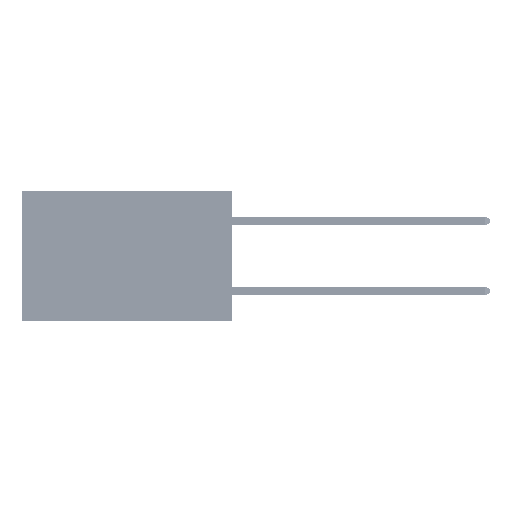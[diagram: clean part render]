
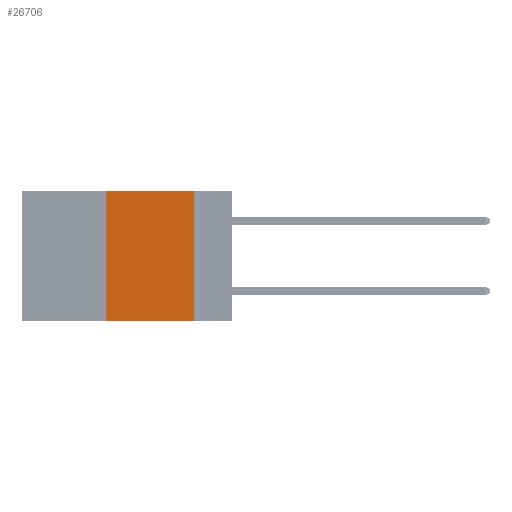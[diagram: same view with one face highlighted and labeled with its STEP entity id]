
A CAD part, left-side view. The second image highlights one B-rep face of the part: STEP entity #26706.
In plain terms, the highlighted planar face has unit normal (-1, 0, 0).
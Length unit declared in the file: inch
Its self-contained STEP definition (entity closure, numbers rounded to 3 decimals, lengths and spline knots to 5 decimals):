
#511 = CARTESIAN_POINT ( 'NONE',  ( 0., 0.6, -0.37 ) ) ;
#1195 = VECTOR ( 'NONE', #3777, 39.37008 ) ;
#1371 = DIRECTION ( 'NONE',  ( 1., 0., 0. ) ) ;
#3777 = DIRECTION ( 'NONE',  ( 0., -1., 0. ) ) ;
#5185 = FACE_OUTER_BOUND ( 'NONE', #28197, .T. ) ;
#6733 = VECTOR ( 'NONE', #9785, 39.37008 ) ;
#6954 = EDGE_CURVE ( 'NONE', #17220, #30719, #17455, .T. ) ;
#7399 = CARTESIAN_POINT ( 'NONE',  ( 0., 0.36, 0. ) ) ;
#9785 = DIRECTION ( 'NONE',  ( 0., 0., -1. ) ) ;
#10021 = DIRECTION ( 'NONE',  ( 0., 0., -1. ) ) ;
#10980 = DIRECTION ( 'NONE',  ( 0., 0., 1. ) ) ;
#13356 = EDGE_CURVE ( 'NONE', #19808, #17220, #43377, .T. ) ;
#15322 = VECTOR ( 'NONE', #10980, 39.37008 ) ;
#15747 = EDGE_CURVE ( 'NONE', #37429, #30719, #19131, .T. ) ;
#16372 = AXIS2_PLACEMENT_3D ( 'NONE', #19773, #1371, #10021 ) ;
#17131 = ORIENTED_EDGE ( 'NONE', *, *, #15747, .T. ) ;
#17220 = VERTEX_POINT ( 'NONE', #33441 ) ;
#17455 = LINE ( 'NONE', #29238, #6733 ) ;
#19131 = LINE ( 'NONE', #511, #46562 ) ;
#19773 = CARTESIAN_POINT ( 'NONE',  ( 0., 0.6, 0. ) ) ;
#19808 = VERTEX_POINT ( 'NONE', #44841 ) ;
#21974 = LINE ( 'NONE', #7399, #15322 ) ;
#24375 = ORIENTED_EDGE ( 'NONE', *, *, #6954, .F. ) ;
#26706 = ADVANCED_FACE ( 'NONE', ( #5185 ), #36378, .F. ) ;
#27159 = ORIENTED_EDGE ( 'NONE', *, *, #13356, .F. ) ;
#28197 = EDGE_LOOP ( 'NONE', ( #24375, #27159, #46384, #17131 ) ) ;
#28507 = CARTESIAN_POINT ( 'NONE',  ( 0., 0.11, -0.37 ) ) ;
#29238 = CARTESIAN_POINT ( 'NONE',  ( 0., 0.11, 0. ) ) ;
#30719 = VERTEX_POINT ( 'NONE', #28507 ) ;
#33441 = CARTESIAN_POINT ( 'NONE',  ( 0., 0.11, 0. ) ) ;
#34760 = DIRECTION ( 'NONE',  ( 0., -1., 0. ) ) ;
#36378 = PLANE ( 'NONE',  #16372 ) ;
#37429 = VERTEX_POINT ( 'NONE', #39978 ) ;
#38780 = CARTESIAN_POINT ( 'NONE',  ( 0., 0.6, 0. ) ) ;
#39978 = CARTESIAN_POINT ( 'NONE',  ( 0., 0.36, -0.37 ) ) ;
#43377 = LINE ( 'NONE', #38780, #1195 ) ;
#44841 = CARTESIAN_POINT ( 'NONE',  ( 0., 0.36, 0. ) ) ;
#46381 = EDGE_CURVE ( 'NONE', #37429, #19808, #21974, .T. ) ;
#46384 = ORIENTED_EDGE ( 'NONE', *, *, #46381, .F. ) ;
#46562 = VECTOR ( 'NONE', #34760, 39.37008 ) ;
